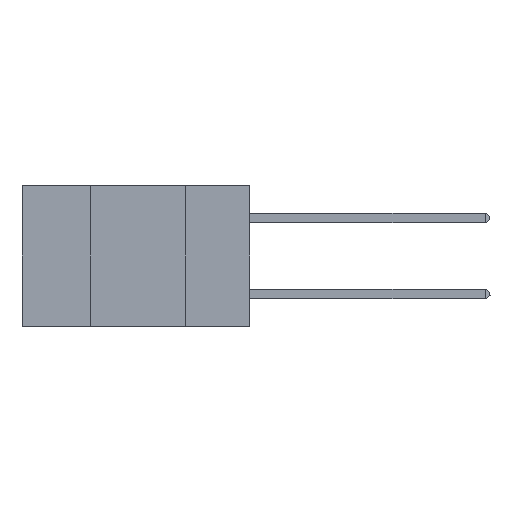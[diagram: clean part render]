
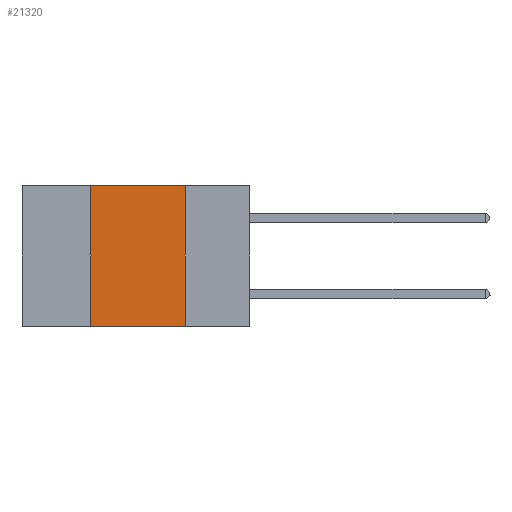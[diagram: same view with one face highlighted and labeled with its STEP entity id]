
A CAD part, left-side view. The second image highlights one B-rep face of the part: STEP entity #21320.
In plain terms, the highlighted planar face has unit normal (-1, 0, 0).
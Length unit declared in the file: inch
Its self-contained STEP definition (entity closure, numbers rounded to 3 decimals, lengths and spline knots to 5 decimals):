
#1660 = PLANE ( 'NONE',  #34263 ) ;
#2146 = DIRECTION ( 'NONE',  ( 0., 0., 1. ) ) ;
#5218 = LINE ( 'NONE', #29694, #33894 ) ;
#6619 = CARTESIAN_POINT ( 'NONE',  ( 0., 0.6, 0. ) ) ;
#6851 = FACE_OUTER_BOUND ( 'NONE', #26845, .T. ) ;
#7572 = LINE ( 'NONE', #13233, #12038 ) ;
#9645 = DIRECTION ( 'NONE',  ( 0., 0., -1. ) ) ;
#10470 = CARTESIAN_POINT ( 'NONE',  ( 0., 0.6, -0.37 ) ) ;
#11240 = ORIENTED_EDGE ( 'NONE', *, *, #33986, .F. ) ;
#11761 = CARTESIAN_POINT ( 'NONE',  ( 0., 0.42, -0.37 ) ) ;
#12038 = VECTOR ( 'NONE', #2146, 39.37008 ) ;
#13233 = CARTESIAN_POINT ( 'NONE',  ( 0., 0.42, 0. ) ) ;
#15208 = DIRECTION ( 'NONE',  ( 0., -1., 0. ) ) ;
#16336 = DIRECTION ( 'NONE',  ( 0., -1., 0. ) ) ;
#17627 = EDGE_CURVE ( 'NONE', #24004, #26931, #7572, .T. ) ;
#18654 = CARTESIAN_POINT ( 'NONE',  ( 0., 0.17, 0. ) ) ;
#19271 = CARTESIAN_POINT ( 'NONE',  ( 0., 0.17, -0.37 ) ) ;
#20953 = EDGE_CURVE ( 'NONE', #24004, #35774, #30643, .T. ) ;
#21320 = ADVANCED_FACE ( 'NONE', ( #6851 ), #1660, .F. ) ;
#21806 = ORIENTED_EDGE ( 'NONE', *, *, #17627, .F. ) ;
#22036 = VERTEX_POINT ( 'NONE', #18654 ) ;
#22936 = ORIENTED_EDGE ( 'NONE', *, *, #26918, .F. ) ;
#24004 = VERTEX_POINT ( 'NONE', #11761 ) ;
#26845 = EDGE_LOOP ( 'NONE', ( #22936, #11240, #21806, #36918 ) ) ;
#26918 = EDGE_CURVE ( 'NONE', #22036, #35774, #5218, .T. ) ;
#26931 = VERTEX_POINT ( 'NONE', #35466 ) ;
#27367 = DIRECTION ( 'NONE',  ( 1., 0., 0. ) ) ;
#27614 = CARTESIAN_POINT ( 'NONE',  ( 0., 0.6, 0. ) ) ;
#28821 = LINE ( 'NONE', #6619, #29793 ) ;
#29694 = CARTESIAN_POINT ( 'NONE',  ( 0., 0.17, 0. ) ) ;
#29793 = VECTOR ( 'NONE', #15208, 39.37008 ) ;
#30534 = DIRECTION ( 'NONE',  ( 0., 0., -1. ) ) ;
#30643 = LINE ( 'NONE', #10470, #35584 ) ;
#33894 = VECTOR ( 'NONE', #9645, 39.37008 ) ;
#33986 = EDGE_CURVE ( 'NONE', #26931, #22036, #28821, .T. ) ;
#34263 = AXIS2_PLACEMENT_3D ( 'NONE', #27614, #27367, #30534 ) ;
#35466 = CARTESIAN_POINT ( 'NONE',  ( 0., 0.42, 0. ) ) ;
#35584 = VECTOR ( 'NONE', #16336, 39.37008 ) ;
#35774 = VERTEX_POINT ( 'NONE', #19271 ) ;
#36918 = ORIENTED_EDGE ( 'NONE', *, *, #20953, .T. ) ;
